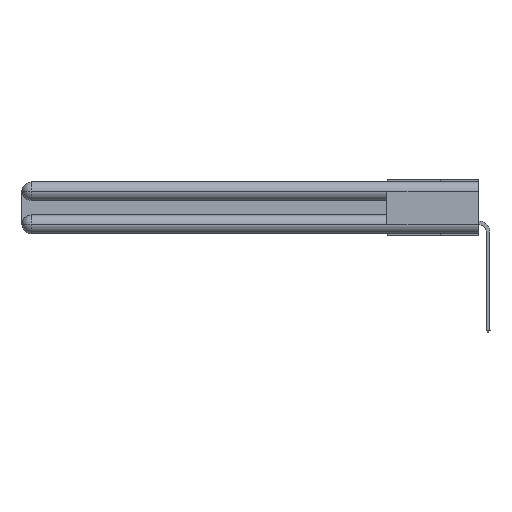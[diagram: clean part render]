
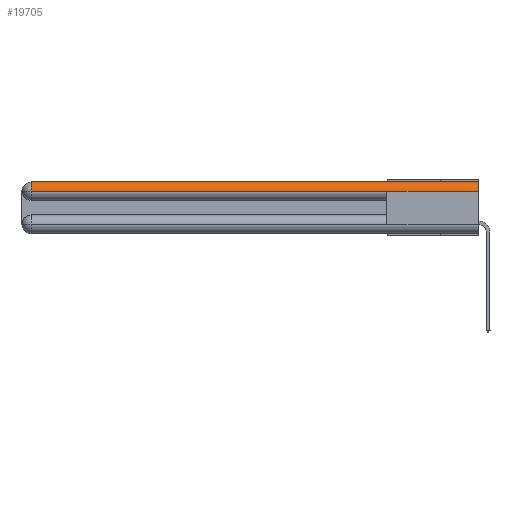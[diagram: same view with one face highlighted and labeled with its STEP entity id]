
A CAD part, left-side view. The second image highlights one B-rep face of the part: STEP entity #19705.
In plain terms, the highlighted cylindrical face has radius 1.562 mm (diameter 3.124 mm), a partial arc.
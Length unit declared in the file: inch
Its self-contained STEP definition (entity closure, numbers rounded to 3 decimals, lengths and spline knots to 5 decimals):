
#374 = LINE ( 'NONE', #14445, #6894 ) ;
#1580 = ORIENTED_EDGE ( 'NONE', *, *, #15202, .F. ) ;
#3430 = AXIS2_PLACEMENT_3D ( 'NONE', #8203, #21286, #23830 ) ;
#4149 = EDGE_LOOP ( 'NONE', ( #1580, #28978, #26341, #25709, #32888 ) ) ;
#5652 = EDGE_CURVE ( 'NONE', #31038, #20823, #374, .T. ) ;
#6223 = EDGE_CURVE ( 'NONE', #7190, #22122, #26986, .T. ) ;
#6894 = VECTOR ( 'NONE', #33129, 39.37008 ) ;
#7190 = VERTEX_POINT ( 'NONE', #20128 ) ;
#7358 = CARTESIAN_POINT ( 'NONE',  ( 0.0615, 0., -0.0615 ) ) ;
#8019 = CARTESIAN_POINT ( 'NONE',  ( 0., 0.6, -0.0615 ) ) ;
#8203 = CARTESIAN_POINT ( 'NONE',  ( 0.0615, 0., -0.0615 ) ) ;
#9600 = LINE ( 'NONE', #25022, #22749 ) ;
#9975 = DIRECTION ( 'NONE',  ( 0., 0., 1. ) ) ;
#10387 = DIRECTION ( 'NONE',  ( 0., -1., 0. ) ) ;
#10549 = DIRECTION ( 'NONE',  ( 0., 1., 0. ) ) ;
#10981 = CYLINDRICAL_SURFACE ( 'NONE', #19510, 0.0615 ) ;
#14445 = CARTESIAN_POINT ( 'NONE',  ( 0., 3., -0.0615 ) ) ;
#14956 = CARTESIAN_POINT ( 'NONE',  ( 0., 2.94, -0.0615 ) ) ;
#15202 = EDGE_CURVE ( 'NONE', #19521, #7190, #9600, .T. ) ;
#16181 = CARTESIAN_POINT ( 'NONE',  ( 0.0615, 2.94, 0. ) ) ;
#17099 = FACE_OUTER_BOUND ( 'NONE', #4149, .T. ) ;
#17696 = EDGE_CURVE ( 'NONE', #22122, #20823, #23872, .T. ) ;
#18053 = CIRCLE ( 'NONE', #18762, 0.0615 ) ;
#18762 = AXIS2_PLACEMENT_3D ( 'NONE', #31840, #10387, #21062 ) ;
#19510 = AXIS2_PLACEMENT_3D ( 'NONE', #7358, #23068, #9975 ) ;
#19521 = VERTEX_POINT ( 'NONE', #16181 ) ;
#19705 = ADVANCED_FACE ( 'NONE', ( #17099 ), #10981, .T. ) ;
#20128 = CARTESIAN_POINT ( 'NONE',  ( 0.0615, 0., 0. ) ) ;
#20217 = CARTESIAN_POINT ( 'NONE',  ( 0., 0., -0.0615 ) ) ;
#20823 = VERTEX_POINT ( 'NONE', #8019 ) ;
#21062 = DIRECTION ( 'NONE',  ( 0., 0., 1. ) ) ;
#21286 = DIRECTION ( 'NONE',  ( 0., -1., 0. ) ) ;
#22122 = VERTEX_POINT ( 'NONE', #20217 ) ;
#22749 = VECTOR ( 'NONE', #27636, 39.37008 ) ;
#23068 = DIRECTION ( 'NONE',  ( 0., 1., 0. ) ) ;
#23830 = DIRECTION ( 'NONE',  ( 1., 0., 0. ) ) ;
#23872 = LINE ( 'NONE', #29127, #32466 ) ;
#25022 = CARTESIAN_POINT ( 'NONE',  ( 0.0615, 0., 0. ) ) ;
#25709 = ORIENTED_EDGE ( 'NONE', *, *, #17696, .F. ) ;
#26341 = ORIENTED_EDGE ( 'NONE', *, *, #5652, .T. ) ;
#26986 = CIRCLE ( 'NONE', #3430, 0.0615 ) ;
#27047 = EDGE_CURVE ( 'NONE', #19521, #31038, #18053, .T. ) ;
#27636 = DIRECTION ( 'NONE',  ( 0., -1., 0. ) ) ;
#28978 = ORIENTED_EDGE ( 'NONE', *, *, #27047, .T. ) ;
#29127 = CARTESIAN_POINT ( 'NONE',  ( 0., 3., -0.0615 ) ) ;
#31038 = VERTEX_POINT ( 'NONE', #14956 ) ;
#31840 = CARTESIAN_POINT ( 'NONE',  ( 0.0615, 2.94, -0.0615 ) ) ;
#32466 = VECTOR ( 'NONE', #10549, 39.37008 ) ;
#32888 = ORIENTED_EDGE ( 'NONE', *, *, #6223, .F. ) ;
#33129 = DIRECTION ( 'NONE',  ( 0., -1., 0. ) ) ;
